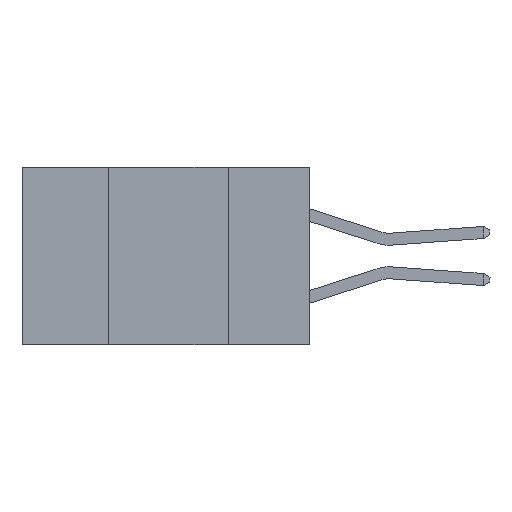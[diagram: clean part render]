
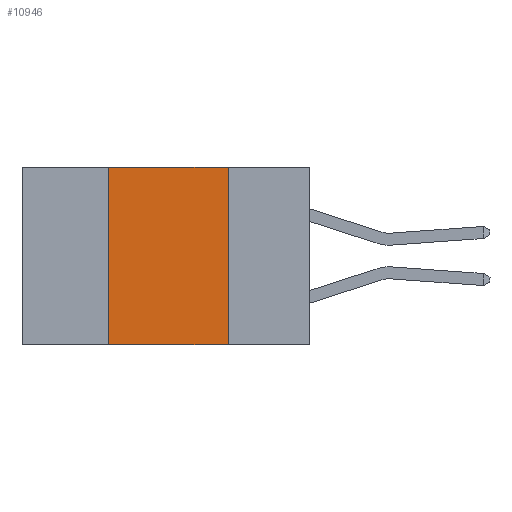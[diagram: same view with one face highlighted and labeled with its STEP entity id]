
A CAD part, left-side view. The second image highlights one B-rep face of the part: STEP entity #10946.
In plain terms, the highlighted planar face has unit normal (-1, 0, 0).
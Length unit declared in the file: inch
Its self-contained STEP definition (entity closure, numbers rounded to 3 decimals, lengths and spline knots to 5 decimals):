
#60 = CARTESIAN_POINT ( 'NONE',  ( 0., 0.42, 0. ) ) ;
#789 = LINE ( 'NONE', #60, #5898 ) ;
#2956 = VERTEX_POINT ( 'NONE', #26124 ) ;
#4014 = ORIENTED_EDGE ( 'NONE', *, *, #12000, .F. ) ;
#5832 = CARTESIAN_POINT ( 'NONE',  ( 0., 0.42, 0. ) ) ;
#5898 = VECTOR ( 'NONE', #7654, 39.37008 ) ;
#6893 = CARTESIAN_POINT ( 'NONE',  ( 0., 0.6, -0.37 ) ) ;
#6974 = EDGE_CURVE ( 'NONE', #10000, #2956, #27582, .T. ) ;
#7561 = CARTESIAN_POINT ( 'NONE',  ( 0., 0.17, 0. ) ) ;
#7654 = DIRECTION ( 'NONE',  ( 0., 0., 1. ) ) ;
#7949 = LINE ( 'NONE', #6893, #13797 ) ;
#8163 = VERTEX_POINT ( 'NONE', #5832 ) ;
#10000 = VERTEX_POINT ( 'NONE', #7561 ) ;
#10020 = VERTEX_POINT ( 'NONE', #12572 ) ;
#10946 = ADVANCED_FACE ( 'NONE', ( #29726 ), #23742, .F. ) ;
#11102 = DIRECTION ( 'NONE',  ( 0., 0., -1. ) ) ;
#12000 = EDGE_CURVE ( 'NONE', #10020, #8163, #789, .T. ) ;
#12572 = CARTESIAN_POINT ( 'NONE',  ( 0., 0.42, -0.37 ) ) ;
#13797 = VECTOR ( 'NONE', #19425, 39.37008 ) ;
#14621 = AXIS2_PLACEMENT_3D ( 'NONE', #21162, #26315, #11102 ) ;
#15426 = VECTOR ( 'NONE', #25173, 39.37008 ) ;
#15732 = EDGE_CURVE ( 'NONE', #8163, #10000, #22225, .T. ) ;
#15851 = CARTESIAN_POINT ( 'NONE',  ( 0., 0.17, 0. ) ) ;
#17721 = EDGE_LOOP ( 'NONE', ( #26128, #28503, #4014, #21684 ) ) ;
#18407 = DIRECTION ( 'NONE',  ( 0., 0., -1. ) ) ;
#18743 = EDGE_CURVE ( 'NONE', #10020, #2956, #7949, .T. ) ;
#19425 = DIRECTION ( 'NONE',  ( 0., -1., 0. ) ) ;
#21162 = CARTESIAN_POINT ( 'NONE',  ( 0., 0.6, 0. ) ) ;
#21684 = ORIENTED_EDGE ( 'NONE', *, *, #18743, .T. ) ;
#22225 = LINE ( 'NONE', #27727, #15426 ) ;
#23742 = PLANE ( 'NONE',  #14621 ) ;
#25173 = DIRECTION ( 'NONE',  ( 0., -1., 0. ) ) ;
#25194 = VECTOR ( 'NONE', #18407, 39.37008 ) ;
#26124 = CARTESIAN_POINT ( 'NONE',  ( 0., 0.17, -0.37 ) ) ;
#26128 = ORIENTED_EDGE ( 'NONE', *, *, #6974, .F. ) ;
#26315 = DIRECTION ( 'NONE',  ( 1., 0., 0. ) ) ;
#27582 = LINE ( 'NONE', #15851, #25194 ) ;
#27727 = CARTESIAN_POINT ( 'NONE',  ( 0., 0.6, 0. ) ) ;
#28503 = ORIENTED_EDGE ( 'NONE', *, *, #15732, .F. ) ;
#29726 = FACE_OUTER_BOUND ( 'NONE', #17721, .T. ) ;
